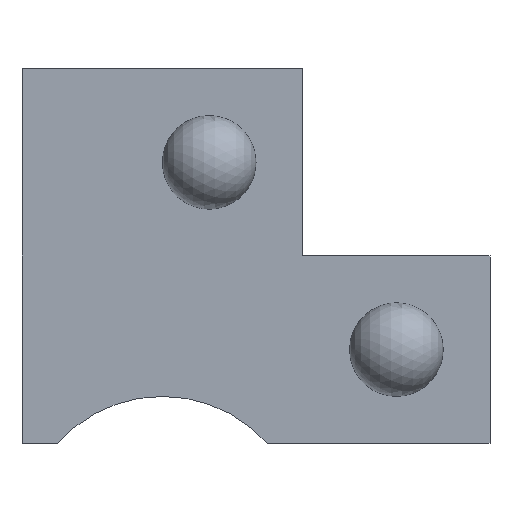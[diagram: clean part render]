
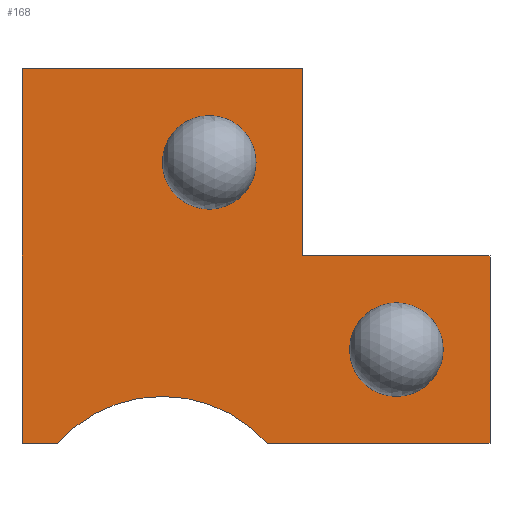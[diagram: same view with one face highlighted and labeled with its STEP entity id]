
A CAD part, left-side view. The second image highlights one B-rep face of the part: STEP entity #168.
In plain terms, the highlighted planar face has unit normal (-1, 0, 0).
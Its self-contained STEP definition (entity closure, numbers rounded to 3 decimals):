
#3 = CARTESIAN_POINT ( 'NONE',  ( 0., 8.09, -15. ) ) ;
#7 = CARTESIAN_POINT ( 'NONE',  ( 0., 10., 5. ) ) ;
#9 = DIRECTION ( 'NONE',  ( 0., 0., -1. ) ) ;
#32 = DIRECTION ( 'NONE',  ( -1., 0., 0. ) ) ;
#34 = CARTESIAN_POINT ( 'NONE',  ( 0., -10., -10. ) ) ;
#41 = PLANE ( 'NONE',  #466 ) ;
#53 = CARTESIAN_POINT ( 'NONE',  ( 0., 10., -15. ) ) ;
#56 = DIRECTION ( 'NONE',  ( 0., 0., -1. ) ) ;
#57 = DIRECTION ( 'NONE',  ( 0., 0., -1. ) ) ;
#66 = ORIENTED_EDGE ( 'NONE', *, *, #532, .F. ) ;
#91 = CARTESIAN_POINT ( 'NONE',  ( 0., 10., -15. ) ) ;
#106 = DIRECTION ( 'NONE',  ( 0., 1., 0. ) ) ;
#111 = CARTESIAN_POINT ( 'NONE',  ( 0., 0., -2.5 ) ) ;
#112 = CARTESIAN_POINT ( 'NONE',  ( 0., 2.5, -20. ) ) ;
#113 = DIRECTION ( 'NONE',  ( -1., 0., 0. ) ) ;
#132 = DIRECTION ( 'NONE',  ( 0., 0., 1. ) ) ;
#133 = CARTESIAN_POINT ( 'NONE',  ( 0., -3.09, -15. ) ) ;
#139 = CARTESIAN_POINT ( 'NONE',  ( 0., -10., -12.5 ) ) ;
#146 = DIRECTION ( 'NONE',  ( -1., 0., 0. ) ) ;
#153 = DIRECTION ( 'NONE',  ( 0., 0., -1. ) ) ;
#157 = DIRECTION ( 'NONE',  ( 1., 0., 0. ) ) ;
#163 = CARTESIAN_POINT ( 'NONE',  ( 0., 0., 5. ) ) ;
#165 = CARTESIAN_POINT ( 'NONE',  ( 0., -15., -5. ) ) ;
#166 = VECTOR ( 'NONE', #219, 1000. ) ;
#168 = ADVANCED_FACE ( 'NONE', ( #313, #321, #323 ), #41, .F. ) ;
#171 = CIRCLE ( 'NONE', #385, 7.5 ) ;
#207 = EDGE_CURVE ( 'NONE', #542, #541, #305, .T. ) ;
#217 = CIRCLE ( 'NONE', #406, 2.5 ) ;
#218 = VECTOR ( 'NONE', #237, 1000. ) ;
#219 = DIRECTION ( 'NONE',  ( 0., 1., 0. ) ) ;
#223 = CARTESIAN_POINT ( 'NONE',  ( 0., 0., 0. ) ) ;
#225 = LINE ( 'NONE', #91, #218 ) ;
#227 = CIRCLE ( 'NONE', #407, 2.5 ) ;
#229 = CARTESIAN_POINT ( 'NONE',  ( 0., 0., 0. ) ) ;
#231 = VECTOR ( 'NONE', #471, 1000. ) ;
#234 = VECTOR ( 'NONE', #57, 1000. ) ;
#235 = CARTESIAN_POINT ( 'NONE',  ( 0., -15., -15. ) ) ;
#237 = DIRECTION ( 'NONE',  ( 0., 0., 1. ) ) ;
#238 = LINE ( 'NONE', #163, #231 ) ;
#240 = VECTOR ( 'NONE', #468, 1000. ) ;
#241 = LINE ( 'NONE', #366, #240 ) ;
#242 = LINE ( 'NONE', #643, #234 ) ;
#244 = CIRCLE ( 'NONE', #408, 7.5 ) ;
#248 = VECTOR ( 'NONE', #9, 1000. ) ;
#250 = LINE ( 'NONE', #235, #248 ) ;
#251 = CIRCLE ( 'NONE', #411, 2.5 ) ;
#269 = VECTOR ( 'NONE', #106, 1000. ) ;
#273 = LINE ( 'NONE', #553, #269 ) ;
#277 = CIRCLE ( 'NONE', #437, 2.5 ) ;
#299 = DIRECTION ( 'NONE',  ( 0., 0., -1. ) ) ;
#300 = DIRECTION ( 'NONE',  ( -1., 0., 0. ) ) ;
#305 = LINE ( 'NONE', #358, #166 ) ;
#313 = FACE_BOUND ( 'NONE', #403, .T. ) ;
#321 = FACE_OUTER_BOUND ( 'NONE', #369, .T. ) ;
#323 = FACE_BOUND ( 'NONE', #502, .T. ) ;
#327 = EDGE_CURVE ( 'NONE', #582, #440, #277, .T. ) ;
#342 = EDGE_CURVE ( 'NONE', #463, #507, #273, .T. ) ;
#355 = CARTESIAN_POINT ( 'NONE',  ( 0., -10., -7.5 ) ) ;
#358 = CARTESIAN_POINT ( 'NONE',  ( 0., -15., -5. ) ) ;
#359 = CARTESIAN_POINT ( 'NONE',  ( 0., -5., 5. ) ) ;
#366 = CARTESIAN_POINT ( 'NONE',  ( 0., 5., -15. ) ) ;
#369 = EDGE_LOOP ( 'NONE', ( #509, #384, #66, #552, #413, #629, #585, #444, #656 ) ) ;
#371 = VERTEX_POINT ( 'NONE', #355 ) ;
#384 = ORIENTED_EDGE ( 'NONE', *, *, #608, .F. ) ;
#385 = AXIS2_PLACEMENT_3D ( 'NONE', #614, #146, #661 ) ;
#403 = EDGE_LOOP ( 'NONE', ( #641, #618 ) ) ;
#406 = AXIS2_PLACEMENT_3D ( 'NONE', #469, #113, #563 ) ;
#407 = AXIS2_PLACEMENT_3D ( 'NONE', #34, #300, #56 ) ;
#408 = AXIS2_PLACEMENT_3D ( 'NONE', #112, #560, #132 ) ;
#411 = AXIS2_PLACEMENT_3D ( 'NONE', #229, #32, #299 ) ;
#413 = ORIENTED_EDGE ( 'NONE', *, *, #536, .F. ) ;
#437 = AXIS2_PLACEMENT_3D ( 'NONE', #631, #545, #455 ) ;
#440 = VERTEX_POINT ( 'NONE', #630 ) ;
#444 = ORIENTED_EDGE ( 'NONE', *, *, #538, .F. ) ;
#455 = DIRECTION ( 'NONE',  ( 0., 0., -1. ) ) ;
#463 = VERTEX_POINT ( 'NONE', #3 ) ;
#466 = AXIS2_PLACEMENT_3D ( 'NONE', #223, #157, #153 ) ;
#468 = DIRECTION ( 'NONE',  ( 0., 1., 0. ) ) ;
#469 = CARTESIAN_POINT ( 'NONE',  ( 0., -10., -10. ) ) ;
#471 = DIRECTION ( 'NONE',  ( 0., -1., 0. ) ) ;
#492 = ORIENTED_EDGE ( 'NONE', *, *, #555, .F. ) ;
#502 = EDGE_LOOP ( 'NONE', ( #606, #492 ) ) ;
#507 = VERTEX_POINT ( 'NONE', #53 ) ;
#509 = ORIENTED_EDGE ( 'NONE', *, *, #342, .F. ) ;
#519 = CARTESIAN_POINT ( 'NONE',  ( 0., 2.5, -12.5 ) ) ;
#521 = VERTEX_POINT ( 'NONE', #623 ) ;
#529 = EDGE_CURVE ( 'NONE', #440, #582, #251, .T. ) ;
#530 = VERTEX_POINT ( 'NONE', #359 ) ;
#532 = EDGE_CURVE ( 'NONE', #559, #628, #244, .T. ) ;
#534 = VERTEX_POINT ( 'NONE', #7 ) ;
#535 = EDGE_CURVE ( 'NONE', #521, #559, #241, .T. ) ;
#536 = EDGE_CURVE ( 'NONE', #542, #521, #250, .T. ) ;
#537 = EDGE_CURVE ( 'NONE', #530, #541, #242, .T. ) ;
#538 = EDGE_CURVE ( 'NONE', #534, #530, #238, .T. ) ;
#541 = VERTEX_POINT ( 'NONE', #647 ) ;
#542 = VERTEX_POINT ( 'NONE', #165 ) ;
#543 = EDGE_CURVE ( 'NONE', #507, #534, #225, .T. ) ;
#545 = DIRECTION ( 'NONE',  ( -1., 0., 0. ) ) ;
#549 = EDGE_CURVE ( 'NONE', #599, #371, #227, .T. ) ;
#552 = ORIENTED_EDGE ( 'NONE', *, *, #535, .F. ) ;
#553 = CARTESIAN_POINT ( 'NONE',  ( 0., 5., -15. ) ) ;
#555 = EDGE_CURVE ( 'NONE', #371, #599, #217, .T. ) ;
#559 = VERTEX_POINT ( 'NONE', #133 ) ;
#560 = DIRECTION ( 'NONE',  ( -1., 0., 0. ) ) ;
#563 = DIRECTION ( 'NONE',  ( 0., 0., -1. ) ) ;
#582 = VERTEX_POINT ( 'NONE', #111 ) ;
#585 = ORIENTED_EDGE ( 'NONE', *, *, #537, .F. ) ;
#599 = VERTEX_POINT ( 'NONE', #139 ) ;
#606 = ORIENTED_EDGE ( 'NONE', *, *, #549, .F. ) ;
#608 = EDGE_CURVE ( 'NONE', #628, #463, #171, .T. ) ;
#614 = CARTESIAN_POINT ( 'NONE',  ( 0., 2.5, -20. ) ) ;
#618 = ORIENTED_EDGE ( 'NONE', *, *, #529, .F. ) ;
#623 = CARTESIAN_POINT ( 'NONE',  ( 0., -15., -15. ) ) ;
#628 = VERTEX_POINT ( 'NONE', #519 ) ;
#629 = ORIENTED_EDGE ( 'NONE', *, *, #207, .T. ) ;
#630 = CARTESIAN_POINT ( 'NONE',  ( 0., 0., 2.5 ) ) ;
#631 = CARTESIAN_POINT ( 'NONE',  ( 0., 0., 0. ) ) ;
#641 = ORIENTED_EDGE ( 'NONE', *, *, #327, .F. ) ;
#643 = CARTESIAN_POINT ( 'NONE',  ( 0., -5., 0. ) ) ;
#647 = CARTESIAN_POINT ( 'NONE',  ( 0., -5., -5. ) ) ;
#656 = ORIENTED_EDGE ( 'NONE', *, *, #543, .F. ) ;
#661 = DIRECTION ( 'NONE',  ( 0., 0., 1. ) ) ;
